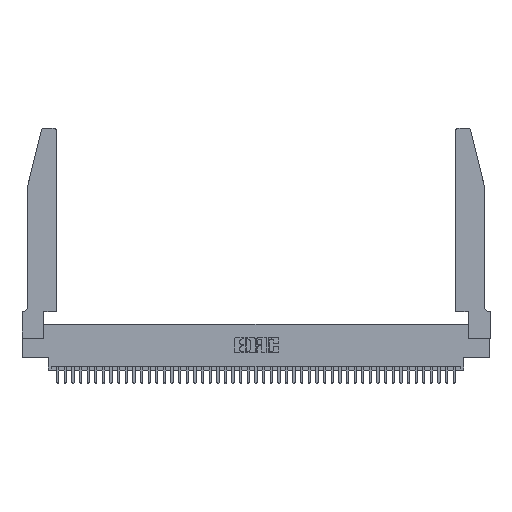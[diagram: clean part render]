
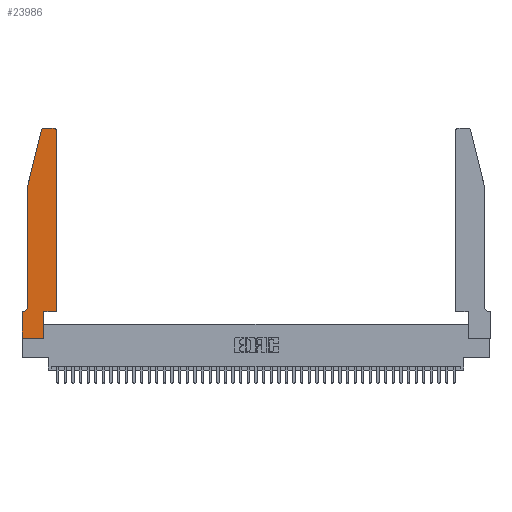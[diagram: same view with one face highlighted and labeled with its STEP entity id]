
A CAD part, top view. The second image highlights one B-rep face of the part: STEP entity #23986.
In plain terms, the highlighted planar face has unit normal (0, 0, 1).
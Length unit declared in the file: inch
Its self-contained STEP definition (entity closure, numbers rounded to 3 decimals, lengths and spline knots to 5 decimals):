
#70 = CARTESIAN_POINT ( 'NONE',  ( 0.2865, 0.35, 0.37 ) ) ;
#85 = AXIS2_PLACEMENT_3D ( 'NONE', #18716, #43003, #22255 ) ;
#89 = ORIENTED_EDGE ( 'NONE', *, *, #14636, .T. ) ;
#568 = VECTOR ( 'NONE', #42471, 39.37008 ) ;
#687 = CARTESIAN_POINT ( 'NONE',  ( 0.0755, 0.35, 0.37 ) ) ;
#1109 = VECTOR ( 'NONE', #27415, 39.37008 ) ;
#1823 = VERTEX_POINT ( 'NONE', #39894 ) ;
#1904 = EDGE_CURVE ( 'NONE', #17955, #13895, #33068, .T. ) ;
#2319 = CARTESIAN_POINT ( 'NONE',  ( 0., 0., 0.37 ) ) ;
#2412 = DIRECTION ( 'NONE',  ( -0.239, -0.971, 0. ) ) ;
#2742 = CARTESIAN_POINT ( 'NONE',  ( 0.284, 2.75, 0.37 ) ) ;
#3111 = DIRECTION ( 'NONE',  ( 1., 0., 0. ) ) ;
#3391 = VERTEX_POINT ( 'NONE', #2742 ) ;
#4236 = CARTESIAN_POINT ( 'NONE',  ( 0.4505, 2.72, 0.37 ) ) ;
#4309 = VERTEX_POINT ( 'NONE', #42749 ) ;
#5267 = ORIENTED_EDGE ( 'NONE', *, *, #38544, .T. ) ;
#5423 = DIRECTION ( 'NONE',  ( 0., 1., 0. ) ) ;
#6330 = VERTEX_POINT ( 'NONE', #39976 ) ;
#7284 = CARTESIAN_POINT ( 'NONE',  ( 0.2605, 2.75, 0.37 ) ) ;
#7955 = LINE ( 'NONE', #2319, #43940 ) ;
#8918 = CARTESIAN_POINT ( 'NONE',  ( 0.4505, 0.35, 0.37 ) ) ;
#9814 = LINE ( 'NONE', #687, #568 ) ;
#10781 = EDGE_CURVE ( 'NONE', #26322, #15236, #40177, .T. ) ;
#10870 = CARTESIAN_POINT ( 'NONE',  ( 0.4205, 2.72, 0.37 ) ) ;
#12808 = ORIENTED_EDGE ( 'NONE', *, *, #36799, .T. ) ;
#12920 = VERTEX_POINT ( 'NONE', #17139 ) ;
#13169 = DIRECTION ( 'NONE',  ( 0., 0., 1. ) ) ;
#13288 = EDGE_LOOP ( 'NONE', ( #37437, #20536, #12808, #14928, #20922, #5267, #32582, #89, #24881, #31922, #18851, #31347 ) ) ;
#13674 = EDGE_CURVE ( 'NONE', #12920, #17955, #17036, .T. ) ;
#13895 = VERTEX_POINT ( 'NONE', #15209 ) ;
#14287 = CIRCLE ( 'NONE', #43908, 0.03 ) ;
#14422 = DIRECTION ( 'NONE',  ( 1., 0., 0. ) ) ;
#14464 = CARTESIAN_POINT ( 'NONE',  ( 0.0755, 0.42, 0.37 ) ) ;
#14636 = EDGE_CURVE ( 'NONE', #35999, #12920, #7955, .T. ) ;
#14928 = ORIENTED_EDGE ( 'NONE', *, *, #18078, .T. ) ;
#15209 = CARTESIAN_POINT ( 'NONE',  ( 0.4505, 0.35, 0.37 ) ) ;
#15236 = VERTEX_POINT ( 'NONE', #33501 ) ;
#15998 = DIRECTION ( 'NONE',  ( 1., 0., 0. ) ) ;
#16034 = LINE ( 'NONE', #8918, #33475 ) ;
#16132 = VERTEX_POINT ( 'NONE', #30860 ) ;
#16389 = DIRECTION ( 'NONE',  ( 1., 0., 0. ) ) ;
#16867 = CARTESIAN_POINT ( 'NONE',  ( 0.0755, 2., 0.37 ) ) ;
#17036 = LINE ( 'NONE', #70, #34466 ) ;
#17091 = LINE ( 'NONE', #37813, #24222 ) ;
#17139 = CARTESIAN_POINT ( 'NONE',  ( 0.2865, 0., 0.37 ) ) ;
#17748 = AXIS2_PLACEMENT_3D ( 'NONE', #41358, #24089, #3111 ) ;
#17955 = VERTEX_POINT ( 'NONE', #24653 ) ;
#18078 = EDGE_CURVE ( 'NONE', #6330, #26322, #19765, .T. ) ;
#18716 = CARTESIAN_POINT ( 'NONE',  ( 0.0055, 0.42, 0.37 ) ) ;
#18851 = ORIENTED_EDGE ( 'NONE', *, *, #37302, .T. ) ;
#19540 = CARTESIAN_POINT ( 'NONE',  ( 0.4505, 0.35, 0.37 ) ) ;
#19765 = LINE ( 'NONE', #16867, #1109 ) ;
#20536 = ORIENTED_EDGE ( 'NONE', *, *, #28930, .T. ) ;
#20922 = ORIENTED_EDGE ( 'NONE', *, *, #10781, .T. ) ;
#22255 = DIRECTION ( 'NONE',  ( -1., 0., 0. ) ) ;
#23986 = ADVANCED_FACE ( 'NONE', ( #34635 ), #44832, .T. ) ;
#24057 = DIRECTION ( 'NONE',  ( 0., -1., 0. ) ) ;
#24089 = DIRECTION ( 'NONE',  ( 0., 0., 1. ) ) ;
#24222 = VECTOR ( 'NONE', #24057, 39.37008 ) ;
#24331 = EDGE_CURVE ( 'NONE', #4309, #3391, #30814, .T. ) ;
#24653 = CARTESIAN_POINT ( 'NONE',  ( 0.2865, 0.35, 0.37 ) ) ;
#24881 = ORIENTED_EDGE ( 'NONE', *, *, #13674, .T. ) ;
#26322 = VERTEX_POINT ( 'NONE', #14464 ) ;
#27415 = DIRECTION ( 'NONE',  ( 0., -1., 0. ) ) ;
#28930 = EDGE_CURVE ( 'NONE', #3391, #1823, #14287, .T. ) ;
#30814 = LINE ( 'NONE', #7284, #44363 ) ;
#30860 = CARTESIAN_POINT ( 'NONE',  ( 0., 0.35, 0.37 ) ) ;
#31347 = ORIENTED_EDGE ( 'NONE', *, *, #40398, .T. ) ;
#31922 = ORIENTED_EDGE ( 'NONE', *, *, #1904, .T. ) ;
#31957 = VECTOR ( 'NONE', #15998, 39.37008 ) ;
#32582 = ORIENTED_EDGE ( 'NONE', *, *, #37704, .T. ) ;
#33068 = LINE ( 'NONE', #19540, #31957 ) ;
#33475 = VECTOR ( 'NONE', #5423, 39.37008 ) ;
#33501 = CARTESIAN_POINT ( 'NONE',  ( 0.0055, 0.35, 0.37 ) ) ;
#33655 = VERTEX_POINT ( 'NONE', #4236 ) ;
#34096 = CARTESIAN_POINT ( 'NONE',  ( 0.284, 2.72, 0.37 ) ) ;
#34466 = VECTOR ( 'NONE', #41855, 39.37008 ) ;
#34635 = FACE_OUTER_BOUND ( 'NONE', #13288, .T. ) ;
#35213 = DIRECTION ( 'NONE',  ( -1., 0., 0. ) ) ;
#35314 = DIRECTION ( 'NONE',  ( 0., 0., 1. ) ) ;
#35999 = VERTEX_POINT ( 'NONE', #39996 ) ;
#36774 = LINE ( 'NONE', #44141, #44901 ) ;
#36799 = EDGE_CURVE ( 'NONE', #1823, #6330, #36774, .T. ) ;
#37302 = EDGE_CURVE ( 'NONE', #13895, #33655, #16034, .T. ) ;
#37437 = ORIENTED_EDGE ( 'NONE', *, *, #24331, .T. ) ;
#37567 = DIRECTION ( 'NONE',  ( 1., 0., 0. ) ) ;
#37704 = EDGE_CURVE ( 'NONE', #16132, #35999, #17091, .T. ) ;
#37813 = CARTESIAN_POINT ( 'NONE',  ( 0., 0., 0.37 ) ) ;
#38544 = EDGE_CURVE ( 'NONE', #15236, #16132, #9814, .T. ) ;
#39378 = CIRCLE ( 'NONE', #44780, 0.03 ) ;
#39894 = CARTESIAN_POINT ( 'NONE',  ( 0.25487, 2.72718, 0.37 ) ) ;
#39976 = CARTESIAN_POINT ( 'NONE',  ( 0.0755, 2., 0.37 ) ) ;
#39996 = CARTESIAN_POINT ( 'NONE',  ( 0., 0., 0.37 ) ) ;
#40177 = CIRCLE ( 'NONE', #85, 0.07 ) ;
#40398 = EDGE_CURVE ( 'NONE', #33655, #4309, #39378, .T. ) ;
#41358 = CARTESIAN_POINT ( 'NONE',  ( 0., 0.35, 0.37 ) ) ;
#41855 = DIRECTION ( 'NONE',  ( 0., 1., 0. ) ) ;
#42471 = DIRECTION ( 'NONE',  ( -1., 0., 0. ) ) ;
#42749 = CARTESIAN_POINT ( 'NONE',  ( 0.4205, 2.75, 0.37 ) ) ;
#43003 = DIRECTION ( 'NONE',  ( 0., 0., -1. ) ) ;
#43908 = AXIS2_PLACEMENT_3D ( 'NONE', #34096, #13169, #37567 ) ;
#43940 = VECTOR ( 'NONE', #16389, 39.37008 ) ;
#44141 = CARTESIAN_POINT ( 'NONE',  ( 0.0755, 2., 0.37 ) ) ;
#44363 = VECTOR ( 'NONE', #35213, 39.37008 ) ;
#44780 = AXIS2_PLACEMENT_3D ( 'NONE', #10870, #35314, #14422 ) ;
#44832 = PLANE ( 'NONE',  #17748 ) ;
#44901 = VECTOR ( 'NONE', #2412, 39.37008 ) ;
